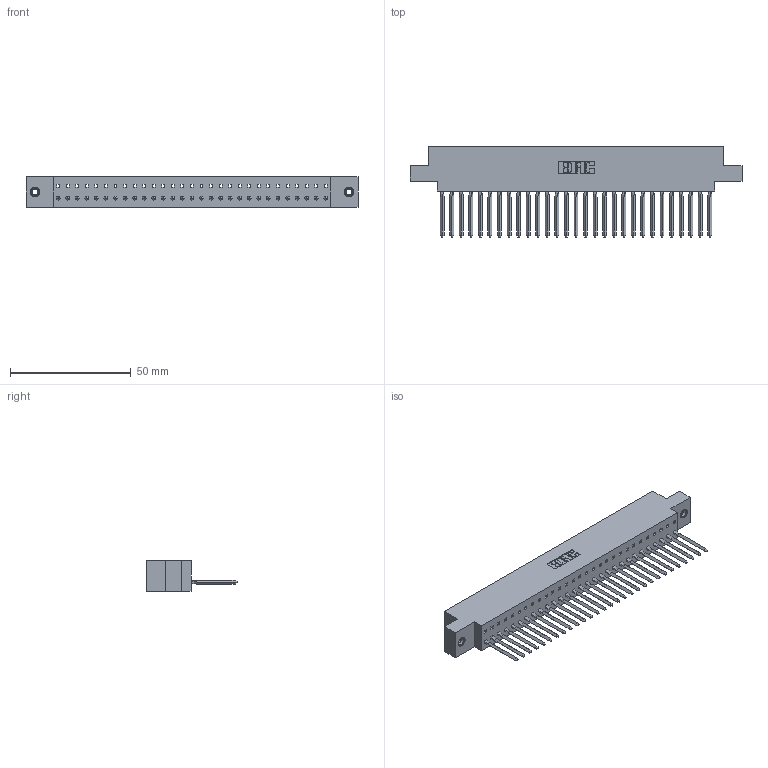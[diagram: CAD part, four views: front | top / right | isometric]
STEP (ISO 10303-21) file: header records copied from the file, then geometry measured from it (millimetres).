
FILE_DESCRIPTION (( 'STEP AP203' ), '1' );
FILE_NAME ('317-029-542-608.STEP', '2020-02-27T19:55:42', ( '' ), ( '' ), 'SwSTEP 2.0', 'SolidWorks 2016', '' );
FILE_SCHEMA (( 'CONFIG_CONTROL_DESIGN' ));
Length unit declared in the file: inch
Products named in the file (4): 345-250-001_345-250-003-102; 317-290-003_542; 317-029-542-608; 317 Part_.156 Dia - TI
Assembly tree (32 placements, depth 2):
  317-029-542-608
    317 Part_.156 Dia - TI
    317-290-003_542  x29
    345-250-001_345-250-003-102  x2
Bounding box: 137.62 x 37.34 x 12.7 mm (x, y, z)
Volume: 20906 mm3; surface area: 25234.8 mm2
Topology: 32 solids, 32 shells, 2337 faces, 6704 edges, 4326 vertices
Faces by surface type: plane 1946, cylinder 259, bspline 116, cone 12, torus 4
Entity records: 43008 total; most frequent: CARTESIAN_POINT 7855, ORIENTED_EDGE 7540, DIRECTION 6346, EDGE_CURVE 3770, LINE 3580, VECTOR 3580, VERTEX_POINT 2504, AXIS2_PLACEMENT_3D 1383
